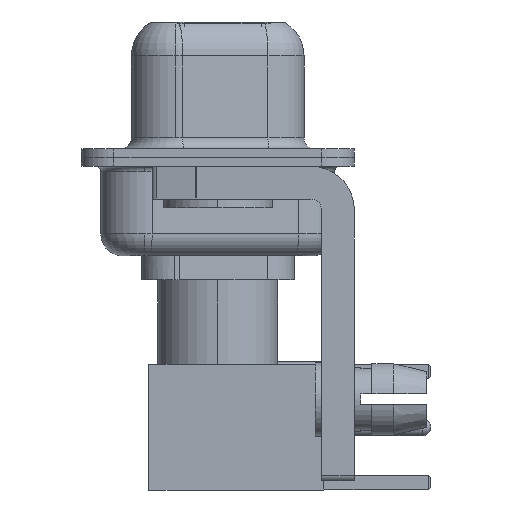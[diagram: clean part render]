
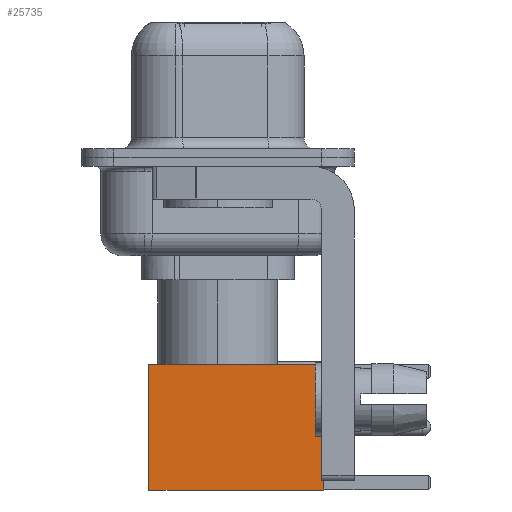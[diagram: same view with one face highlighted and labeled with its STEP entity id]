
A CAD part, left-side view. The second image highlights one B-rep face of the part: STEP entity #25735.
In plain terms, the highlighted face is planar.
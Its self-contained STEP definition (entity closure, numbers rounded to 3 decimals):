
#104 = PLANE ( 'NONE',  #2454 ) ;
#359 = CARTESIAN_POINT ( 'NONE',  ( 2.875, 2.875, 8. ) ) ;
#1053 = ORIENTED_EDGE ( 'NONE', *, *, #22412, .T. ) ;
#1777 = CARTESIAN_POINT ( 'NONE',  ( -2.875, 2.875, 8. ) ) ;
#2454 = AXIS2_PLACEMENT_3D ( 'NONE', #20686, #14884, #8834 ) ;
#2729 = DIRECTION ( 'NONE',  ( 0., 0., -1. ) ) ;
#3272 = VERTEX_POINT ( 'NONE', #1777 ) ;
#4558 = ORIENTED_EDGE ( 'NONE', *, *, #26190, .F. ) ;
#5328 = CARTESIAN_POINT ( 'NONE',  ( -2.875, 2.875, 0. ) ) ;
#5630 = VERTEX_POINT ( 'NONE', #18560 ) ;
#6634 = LINE ( 'NONE', #21176, #11409 ) ;
#6789 = LINE ( 'NONE', #13245, #10108 ) ;
#8741 = EDGE_CURVE ( 'NONE', #3272, #16544, #26224, .T. ) ;
#8834 = DIRECTION ( 'NONE',  ( 0., 0., 1. ) ) ;
#10108 = VECTOR ( 'NONE', #20940, 1000. ) ;
#10779 = CARTESIAN_POINT ( 'NONE',  ( 0., 2.875, 8. ) ) ;
#11409 = VECTOR ( 'NONE', #2729, 1000. ) ;
#11784 = DIRECTION ( 'NONE',  ( 0., 0., -1. ) ) ;
#13061 = LINE ( 'NONE', #10779, #26592 ) ;
#13245 = CARTESIAN_POINT ( 'NONE',  ( 0., 2.875, 0. ) ) ;
#14463 = VERTEX_POINT ( 'NONE', #359 ) ;
#14884 = DIRECTION ( 'NONE',  ( 0., 1., 0. ) ) ;
#16544 = VERTEX_POINT ( 'NONE', #21762 ) ;
#17015 = VECTOR ( 'NONE', #11784, 1000. ) ;
#18560 = CARTESIAN_POINT ( 'NONE',  ( 2.875, 2.875, 0. ) ) ;
#20570 = ORIENTED_EDGE ( 'NONE', *, *, #24244, .T. ) ;
#20686 = CARTESIAN_POINT ( 'NONE',  ( 2.875, 2.875, 0. ) ) ;
#20940 = DIRECTION ( 'NONE',  ( -1., 0., 0. ) ) ;
#21022 = DIRECTION ( 'NONE',  ( -1., 0., 0. ) ) ;
#21176 = CARTESIAN_POINT ( 'NONE',  ( 2.875, 2.875, 0. ) ) ;
#21762 = CARTESIAN_POINT ( 'NONE',  ( -2.875, 2.875, 0. ) ) ;
#22412 = EDGE_CURVE ( 'NONE', #5630, #16544, #6789, .T. ) ;
#24244 = EDGE_CURVE ( 'NONE', #14463, #5630, #6634, .T. ) ;
#24745 = ORIENTED_EDGE ( 'NONE', *, *, #8741, .F. ) ;
#25130 = FACE_OUTER_BOUND ( 'NONE', #25154, .T. ) ;
#25154 = EDGE_LOOP ( 'NONE', ( #20570, #1053, #24745, #4558 ) ) ;
#25735 = ADVANCED_FACE ( 'NONE', ( #25130 ), #104, .T. ) ;
#26190 = EDGE_CURVE ( 'NONE', #14463, #3272, #13061, .T. ) ;
#26224 = LINE ( 'NONE', #5328, #17015 ) ;
#26592 = VECTOR ( 'NONE', #21022, 1000. ) ;
